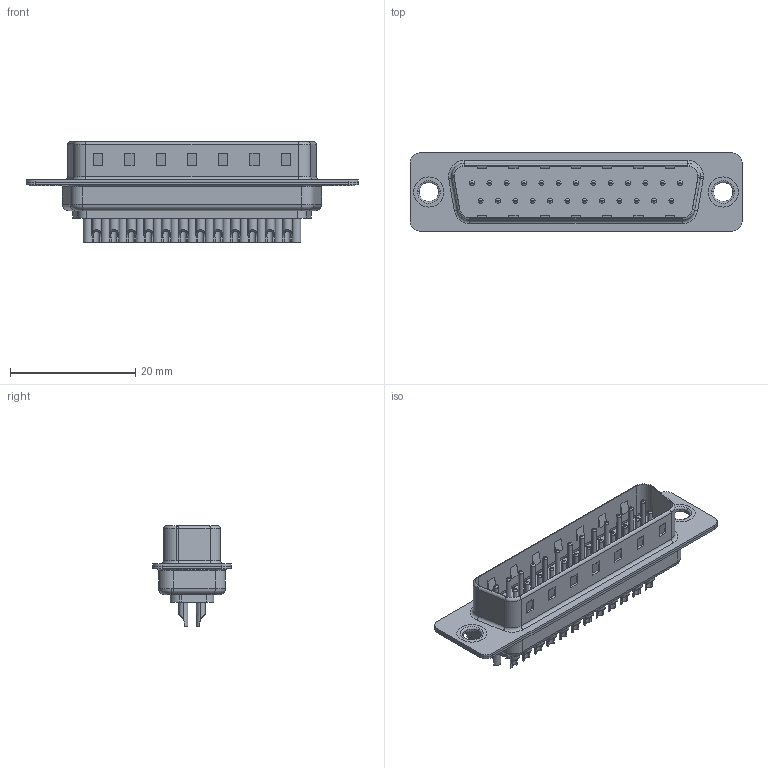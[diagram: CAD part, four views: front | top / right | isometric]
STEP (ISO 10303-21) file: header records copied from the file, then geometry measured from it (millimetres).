
FILE_DESCRIPTION (( 'STEP AP203' ), '1' );
FILE_NAME ('627-M25-322-BN1.STEP', '2021-04-23T15:35:50', ( '' ), ( '' ), 'SwSTEP 2.0', 'SolidWorks 2020', '' );
FILE_SCHEMA (( 'CONFIG_CONTROL_DESIGN' ));
Length unit declared in the file: millimetre
Products named in the file (7): 627M Housing_25 Contacts; 627M Contact Row 2_22; 627-M25-322-BN1; 627M Shell Rear_25 Contacts; 627M Thru Hole Rivet; 627M Shell Front_25 Contacts; 627M Contact Row 1_22
Assembly tree (30 placements, depth 2):
  627-M25-322-BN1
    627M Housing_25 Contacts
    627M Shell Front_25 Contacts
    627M Shell Rear_25 Contacts
    627M Contact Row 1_22  x13
    627M Contact Row 2_22  x12
    627M Thru Hole Rivet  x2
Bounding box: 53.05 x 12.5 x 16.05 mm (x, y, z)
Volume: 2698.2 mm3; surface area: 6932.1 mm2
Topology: 30 solids, 30 shells, 1275 faces, 2975 edges, 1821 vertices
Faces by surface type: cylinder 521, plane 396, torus 308, cone 50
Entity records: 18964 total; most frequent: DIRECTION 3281, CARTESIAN_POINT 3069, ORIENTED_EDGE 2826, EDGE_CURVE 1413, AXIS2_PLACEMENT_3D 1282, VERTEX_POINT 900, EDGE_LOOP 743, VECTOR 717
